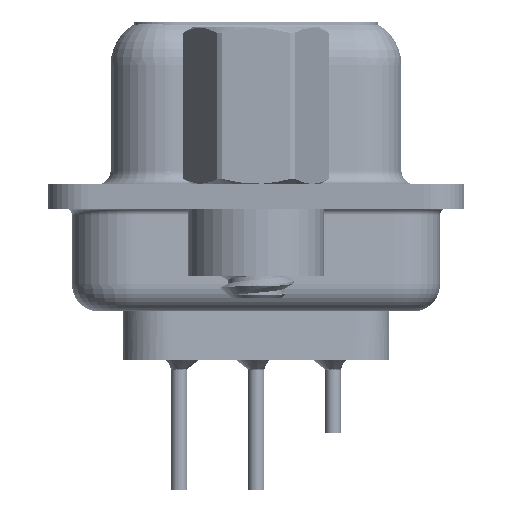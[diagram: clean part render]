
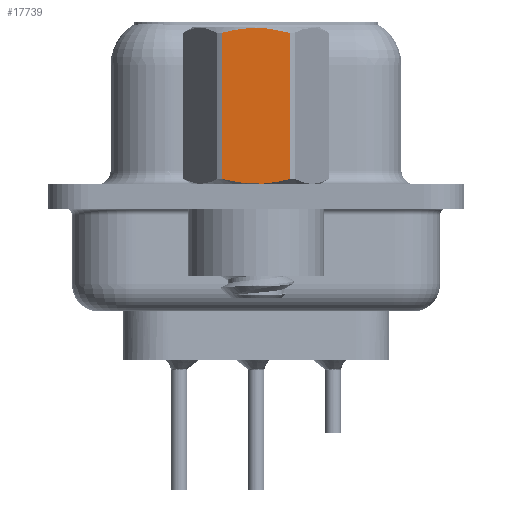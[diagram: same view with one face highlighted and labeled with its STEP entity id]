
A CAD part, left-side view. The second image highlights one B-rep face of the part: STEP entity #17739.
In plain terms, the highlighted planar face has unit normal (-1, 0, 0).
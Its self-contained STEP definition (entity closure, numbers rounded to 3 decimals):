
#1966 = EDGE_CURVE ( 'NONE', #35627, #35214, #41362, .T. ) ;
#4550 = CARTESIAN_POINT ( 'NONE',  ( -2.381, 0.853, 0.549 ) ) ;
#4775 = CARTESIAN_POINT ( 'NONE',  ( -2.381, -0.858, 6.15 ) ) ;
#6333 = VERTEX_POINT ( 'NONE', #38698 ) ;
#7889 = CARTESIAN_POINT ( 'NONE',  ( -2.381, 0.428, 6.215 ) ) ;
#9073 = CARTESIAN_POINT ( 'NONE',  ( -2.381, -1.273, 0.652 ) ) ;
#9469 = EDGE_LOOP ( 'NONE', ( #37321, #41915, #37021, #11240 ) ) ;
#10637 = VECTOR ( 'NONE', #40305, 1000. ) ;
#10966 = VERTEX_POINT ( 'NONE', #33121 ) ;
#11232 = LINE ( 'NONE', #25758, #10637 ) ;
#11240 = ORIENTED_EDGE ( 'NONE', *, *, #17546, .T. ) ;
#11936 = CARTESIAN_POINT ( 'NONE',  ( -2.381, 0.215, 0.468 ) ) ;
#13832 = CARTESIAN_POINT ( 'NONE',  ( -2.381, 1.375, -3.75 ) ) ;
#15247 = CARTESIAN_POINT ( 'NONE',  ( -2.381, -1.066, 6.104 ) ) ;
#15254 = CARTESIAN_POINT ( 'NONE',  ( -2.381, -0.858, 0.55 ) ) ;
#15954 = CARTESIAN_POINT ( 'NONE',  ( -2.381, 1.273, 0.652 ) ) ;
#17546 = EDGE_CURVE ( 'NONE', #10966, #35627, #11232, .T. ) ;
#17739 = ADVANCED_FACE ( 'NONE', ( #28104 ), #46030, .T. ) ;
#20953 = DIRECTION ( 'NONE',  ( 0., -1., 0. ) ) ;
#22880 = CARTESIAN_POINT ( 'NONE',  ( -2.381, -0.215, 0.468 ) ) ;
#25758 = CARTESIAN_POINT ( 'NONE',  ( -2.381, 1.273, 3.792 ) ) ;
#26913 = CARTESIAN_POINT ( 'NONE',  ( -2.381, -0.215, 6.232 ) ) ;
#28099 = VECTOR ( 'NONE', #33342, 1000. ) ;
#28104 = FACE_OUTER_BOUND ( 'NONE', #9469, .T. ) ;
#29764 = CARTESIAN_POINT ( 'NONE',  ( -2.381, 1.273, 6.048 ) ) ;
#29769 = CARTESIAN_POINT ( 'NONE',  ( -2.381, -1.066, 0.596 ) ) ;
#30360 = AXIS2_PLACEMENT_3D ( 'NONE', #13832, #42899, #20953 ) ;
#30475 = CARTESIAN_POINT ( 'NONE',  ( -2.381, -0.432, 6.215 ) ) ;
#30481 = CARTESIAN_POINT ( 'NONE',  ( -2.381, -1.273, 0.652 ) ) ;
#33121 = CARTESIAN_POINT ( 'NONE',  ( -2.381, 1.273, 6.048 ) ) ;
#33342 = DIRECTION ( 'NONE',  ( 0., 0., 1. ) ) ;
#33364 = CARTESIAN_POINT ( 'NONE',  ( -2.381, -1.273, 6.048 ) ) ;
#35214 = VERTEX_POINT ( 'NONE', #9073 ) ;
#35627 = VERTEX_POINT ( 'NONE', #43292 ) ;
#36699 = CARTESIAN_POINT ( 'NONE',  ( -2.381, -0.432, 0.485 ) ) ;
#37021 = ORIENTED_EDGE ( 'NONE', *, *, #39189, .T. ) ;
#37321 = ORIENTED_EDGE ( 'NONE', *, *, #1966, .T. ) ;
#37629 = CARTESIAN_POINT ( 'NONE',  ( -2.381, 0.853, 6.151 ) ) ;
#37636 = CARTESIAN_POINT ( 'NONE',  ( -2.381, 1.065, 0.596 ) ) ;
#38698 = CARTESIAN_POINT ( 'NONE',  ( -2.381, -1.273, 6.048 ) ) ;
#39189 = EDGE_CURVE ( 'NONE', #6333, #10966, #39710, .T. ) ;
#39710 = B_SPLINE_CURVE_WITH_KNOTS ( 'NONE', 3,
 ( #33364, #15247, #4775, #30475, #26913, #44812, #7889, #37629, #41240, #29764 ),
 .UNSPECIFIED., .F., .F.,
 ( 4, 2, 2, 2, 4 ),
 ( 0.001, 0.002, 0.002, 0.003, 0.004 ),
 .UNSPECIFIED. ) ;
#40305 = DIRECTION ( 'NONE',  ( 0., 0., -1. ) ) ;
#41000 = CARTESIAN_POINT ( 'NONE',  ( -2.381, 0.428, 0.485 ) ) ;
#41240 = CARTESIAN_POINT ( 'NONE',  ( -2.381, 1.065, 6.104 ) ) ;
#41362 = B_SPLINE_CURVE_WITH_KNOTS ( 'NONE', 3,
 ( #15954, #37636, #4550, #41000, #11936, #22880, #36699, #15254, #29769, #30481 ),
 .UNSPECIFIED., .F., .F.,
 ( 4, 2, 2, 2, 4 ),
 ( 0.003, 0.003, 0.004, 0.004, 0.005 ),
 .UNSPECIFIED. ) ;
#41915 = ORIENTED_EDGE ( 'NONE', *, *, #45032, .T. ) ;
#42228 = LINE ( 'NONE', #43617, #28099 ) ;
#42899 = DIRECTION ( 'NONE',  ( -1., 0., 0. ) ) ;
#43292 = CARTESIAN_POINT ( 'NONE',  ( -2.381, 1.273, 0.652 ) ) ;
#43617 = CARTESIAN_POINT ( 'NONE',  ( -2.381, -1.273, 3.792 ) ) ;
#44812 = CARTESIAN_POINT ( 'NONE',  ( -2.381, 0.215, 6.232 ) ) ;
#45032 = EDGE_CURVE ( 'NONE', #35214, #6333, #42228, .T. ) ;
#46030 = PLANE ( 'NONE',  #30360 ) ;
